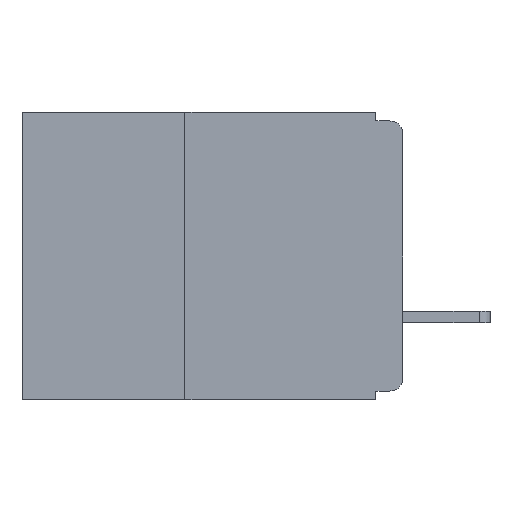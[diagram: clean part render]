
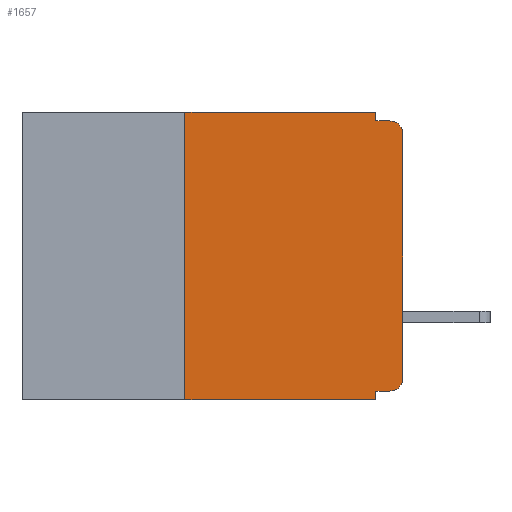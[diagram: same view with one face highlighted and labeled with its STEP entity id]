
A CAD part, left-side view. The second image highlights one B-rep face of the part: STEP entity #1657.
In plain terms, the highlighted planar face has unit normal (-1, 0, 0).
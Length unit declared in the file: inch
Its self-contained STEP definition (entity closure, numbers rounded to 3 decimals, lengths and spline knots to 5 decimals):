
#496 = CARTESIAN_POINT ( 'NONE',  ( 0., 0., -0.305 ) ) ;
#1453 = CIRCLE ( 'NONE', #10228, 0.015 ) ;
#1657 = ADVANCED_FACE ( 'NONE', ( #3321 ), #10910, .F. ) ;
#2008 = VERTEX_POINT ( 'NONE', #496 ) ;
#2012 = CARTESIAN_POINT ( 'NONE',  ( 0., 0.25, -0.33 ) ) ;
#2267 = EDGE_CURVE ( 'NONE', #26460, #27765, #10907, .T. ) ;
#2860 = VERTEX_POINT ( 'NONE', #9883 ) ;
#3201 = AXIS2_PLACEMENT_3D ( 'NONE', #16267, #9598, #16131 ) ;
#3321 = FACE_OUTER_BOUND ( 'NONE', #12782, .T. ) ;
#3618 = CARTESIAN_POINT ( 'NONE',  ( 0., 0.031, 0. ) ) ;
#3784 = EDGE_CURVE ( 'NONE', #27765, #13002, #6195, .T. ) ;
#3865 = ORIENTED_EDGE ( 'NONE', *, *, #27470, .T. ) ;
#3898 = LINE ( 'NONE', #21207, #22251 ) ;
#4378 = CARTESIAN_POINT ( 'NONE',  ( 0., 0., -0.32 ) ) ;
#4937 = EDGE_CURVE ( 'NONE', #15490, #21137, #24505, .T. ) ;
#5225 = CARTESIAN_POINT ( 'NONE',  ( 0., 0.015, -0.305 ) ) ;
#5403 = VECTOR ( 'NONE', #20937, 39.37008 ) ;
#5540 = AXIS2_PLACEMENT_3D ( 'NONE', #5225, #21960, #7692 ) ;
#5758 = CARTESIAN_POINT ( 'NONE',  ( 0., 0.015, -0.025 ) ) ;
#6195 = LINE ( 'NONE', #9607, #12690 ) ;
#6276 = EDGE_CURVE ( 'NONE', #23318, #15490, #18157, .T. ) ;
#6507 = VECTOR ( 'NONE', #21211, 39.37008 ) ;
#6610 = CARTESIAN_POINT ( 'NONE',  ( 0., 0.031, 0. ) ) ;
#6988 = EDGE_CURVE ( 'NONE', #2008, #2860, #3898, .T. ) ;
#7692 = DIRECTION ( 'NONE',  ( 0., 0., -1. ) ) ;
#8172 = EDGE_CURVE ( 'NONE', #27226, #23318, #9906, .T. ) ;
#8183 = ORIENTED_EDGE ( 'NONE', *, *, #6988, .T. ) ;
#8218 = DIRECTION ( 'NONE',  ( 0., 0., -1. ) ) ;
#9373 = DIRECTION ( 'NONE',  ( 0., 0., 1. ) ) ;
#9598 = DIRECTION ( 'NONE',  ( 1., 0., 0. ) ) ;
#9607 = CARTESIAN_POINT ( 'NONE',  ( 0., 0.031, -0.33 ) ) ;
#9711 = DIRECTION ( 'NONE',  ( 0., 0., -1. ) ) ;
#9883 = CARTESIAN_POINT ( 'NONE',  ( 0., 0., -0.025 ) ) ;
#9906 = LINE ( 'NONE', #21052, #15519 ) ;
#10228 = AXIS2_PLACEMENT_3D ( 'NONE', #5758, #22487, #8218 ) ;
#10907 = LINE ( 'NONE', #4378, #17162 ) ;
#10910 = PLANE ( 'NONE',  #3201 ) ;
#11696 = CARTESIAN_POINT ( 'NONE',  ( 0., 0.031, -0.32 ) ) ;
#12274 = EDGE_CURVE ( 'NONE', #14484, #27226, #24763, .T. ) ;
#12354 = DIRECTION ( 'NONE',  ( 0., -1., 0. ) ) ;
#12690 = VECTOR ( 'NONE', #9711, 39.37008 ) ;
#12782 = EDGE_LOOP ( 'NONE', ( #8183, #3865, #21550, #28936, #26523, #26576, #20787, #19407, #13959, #15784 ) ) ;
#12859 = LINE ( 'NONE', #24087, #18351 ) ;
#13002 = VERTEX_POINT ( 'NONE', #18980 ) ;
#13499 = CIRCLE ( 'NONE', #5540, 0.015 ) ;
#13959 = ORIENTED_EDGE ( 'NONE', *, *, #2267, .F. ) ;
#14484 = VERTEX_POINT ( 'NONE', #24095 ) ;
#15490 = VERTEX_POINT ( 'NONE', #18876 ) ;
#15519 = VECTOR ( 'NONE', #16284, 39.37008 ) ;
#15784 = ORIENTED_EDGE ( 'NONE', *, *, #19333, .T. ) ;
#16131 = DIRECTION ( 'NONE',  ( 0., 0., -1. ) ) ;
#16267 = CARTESIAN_POINT ( 'NONE',  ( 0., 0.437, 0. ) ) ;
#16284 = DIRECTION ( 'NONE',  ( 0., -1., 0. ) ) ;
#17162 = VECTOR ( 'NONE', #27060, 39.37008 ) ;
#17619 = EDGE_CURVE ( 'NONE', #14484, #13002, #12859, .T. ) ;
#18157 = LINE ( 'NONE', #6610, #5403 ) ;
#18243 = VECTOR ( 'NONE', #29290, 39.37008 ) ;
#18351 = VECTOR ( 'NONE', #12354, 39.37008 ) ;
#18876 = CARTESIAN_POINT ( 'NONE',  ( 0., 0.031, -0.01 ) ) ;
#18980 = CARTESIAN_POINT ( 'NONE',  ( 0., 0.031, -0.33 ) ) ;
#19333 = EDGE_CURVE ( 'NONE', #26460, #2008, #13499, .T. ) ;
#19407 = ORIENTED_EDGE ( 'NONE', *, *, #3784, .F. ) ;
#20787 = ORIENTED_EDGE ( 'NONE', *, *, #17619, .T. ) ;
#20937 = DIRECTION ( 'NONE',  ( 0., 0., -1. ) ) ;
#21052 = CARTESIAN_POINT ( 'NONE',  ( 0., 0.437, 0. ) ) ;
#21137 = VERTEX_POINT ( 'NONE', #28048 ) ;
#21207 = CARTESIAN_POINT ( 'NONE',  ( 0., 0., 0. ) ) ;
#21211 = DIRECTION ( 'NONE',  ( 0., 0., 1. ) ) ;
#21550 = ORIENTED_EDGE ( 'NONE', *, *, #4937, .F. ) ;
#21960 = DIRECTION ( 'NONE',  ( -1., 0., 0. ) ) ;
#22251 = VECTOR ( 'NONE', #9373, 39.37008 ) ;
#22487 = DIRECTION ( 'NONE',  ( -1., 0., 0. ) ) ;
#23318 = VERTEX_POINT ( 'NONE', #3618 ) ;
#24087 = CARTESIAN_POINT ( 'NONE',  ( 0., 0.437, -0.33 ) ) ;
#24095 = CARTESIAN_POINT ( 'NONE',  ( 0., 0.25, -0.33 ) ) ;
#24505 = LINE ( 'NONE', #29683, #18243 ) ;
#24763 = LINE ( 'NONE', #2012, #6507 ) ;
#25175 = CARTESIAN_POINT ( 'NONE',  ( 0., 0.015, -0.32 ) ) ;
#26460 = VERTEX_POINT ( 'NONE', #25175 ) ;
#26523 = ORIENTED_EDGE ( 'NONE', *, *, #8172, .F. ) ;
#26576 = ORIENTED_EDGE ( 'NONE', *, *, #12274, .F. ) ;
#27060 = DIRECTION ( 'NONE',  ( 0., 1., 0. ) ) ;
#27226 = VERTEX_POINT ( 'NONE', #30077 ) ;
#27470 = EDGE_CURVE ( 'NONE', #2860, #21137, #1453, .T. ) ;
#27765 = VERTEX_POINT ( 'NONE', #11696 ) ;
#28048 = CARTESIAN_POINT ( 'NONE',  ( 0., 0.015, -0.01 ) ) ;
#28936 = ORIENTED_EDGE ( 'NONE', *, *, #6276, .F. ) ;
#29290 = DIRECTION ( 'NONE',  ( 0., -1., 0. ) ) ;
#29683 = CARTESIAN_POINT ( 'NONE',  ( 0., 0., -0.01 ) ) ;
#30077 = CARTESIAN_POINT ( 'NONE',  ( 0., 0.25, 0. ) ) ;
